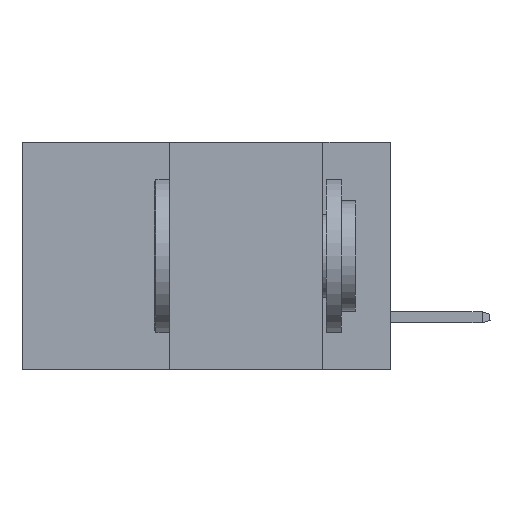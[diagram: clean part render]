
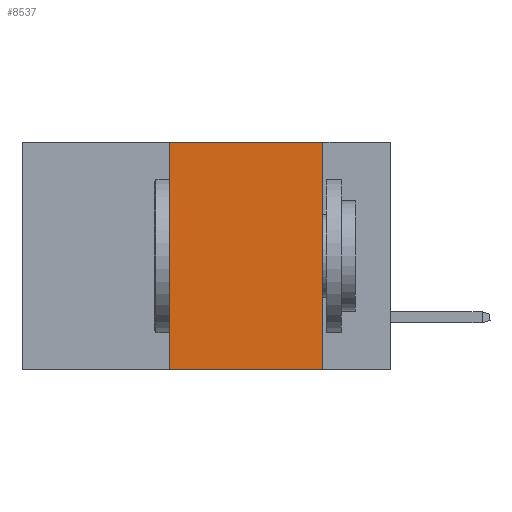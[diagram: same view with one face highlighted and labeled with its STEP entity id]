
A CAD part, left-side view. The second image highlights one B-rep face of the part: STEP entity #8537.
In plain terms, the highlighted planar face has unit normal (-1, 0, 0).
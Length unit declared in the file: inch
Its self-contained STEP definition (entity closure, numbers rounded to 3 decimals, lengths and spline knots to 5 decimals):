
#72 = VECTOR ( 'NONE', #18156, 39.37008 ) ;
#567 = VECTOR ( 'NONE', #1332, 39.37008 ) ;
#1215 = LINE ( 'NONE', #9681, #567 ) ;
#1332 = DIRECTION ( 'NONE',  ( 0., 0., -1. ) ) ;
#2672 = VECTOR ( 'NONE', #10832, 39.37008 ) ;
#2818 = DIRECTION ( 'NONE',  ( 0., -1., 0. ) ) ;
#4038 = ORIENTED_EDGE ( 'NONE', *, *, #9421, .F. ) ;
#4686 = ORIENTED_EDGE ( 'NONE', *, *, #11872, .F. ) ;
#4957 = LINE ( 'NONE', #16290, #72 ) ;
#5154 = VERTEX_POINT ( 'NONE', #15504 ) ;
#6317 = FACE_OUTER_BOUND ( 'NONE', #16492, .T. ) ;
#6521 = CARTESIAN_POINT ( 'NONE',  ( 0., 0.36, 0. ) ) ;
#6741 = CARTESIAN_POINT ( 'NONE',  ( 0., 0.6, -0.37 ) ) ;
#7179 = DIRECTION ( 'NONE',  ( 0., 0., -1. ) ) ;
#7308 = ORIENTED_EDGE ( 'NONE', *, *, #20778, .T. ) ;
#7364 = CARTESIAN_POINT ( 'NONE',  ( 0., 0.36, -0.37 ) ) ;
#8204 = LINE ( 'NONE', #6521, #2672 ) ;
#8537 = ADVANCED_FACE ( 'NONE', ( #6317 ), #19469, .F. ) ;
#9421 = EDGE_CURVE ( 'NONE', #26366, #26115, #8204, .T. ) ;
#9681 = CARTESIAN_POINT ( 'NONE',  ( 0., 0.11, 0. ) ) ;
#10832 = DIRECTION ( 'NONE',  ( 0., 0., 1. ) ) ;
#11872 = EDGE_CURVE ( 'NONE', #17773, #5154, #1215, .T. ) ;
#13207 = CARTESIAN_POINT ( 'NONE',  ( 0., 0.11, 0. ) ) ;
#13343 = CARTESIAN_POINT ( 'NONE',  ( 0., 0.6, 0. ) ) ;
#13422 = DIRECTION ( 'NONE',  ( 1., 0., 0. ) ) ;
#15504 = CARTESIAN_POINT ( 'NONE',  ( 0., 0.11, -0.37 ) ) ;
#15618 = AXIS2_PLACEMENT_3D ( 'NONE', #13343, #13422, #7179 ) ;
#15745 = ORIENTED_EDGE ( 'NONE', *, *, #22935, .F. ) ;
#16290 = CARTESIAN_POINT ( 'NONE',  ( 0., 0.6, 0. ) ) ;
#16492 = EDGE_LOOP ( 'NONE', ( #4686, #15745, #4038, #7308 ) ) ;
#17773 = VERTEX_POINT ( 'NONE', #13207 ) ;
#18156 = DIRECTION ( 'NONE',  ( 0., -1., 0. ) ) ;
#19469 = PLANE ( 'NONE',  #15618 ) ;
#20778 = EDGE_CURVE ( 'NONE', #26366, #5154, #24578, .T. ) ;
#22935 = EDGE_CURVE ( 'NONE', #26115, #17773, #4957, .T. ) ;
#23244 = VECTOR ( 'NONE', #2818, 39.37008 ) ;
#24578 = LINE ( 'NONE', #6741, #23244 ) ;
#25830 = CARTESIAN_POINT ( 'NONE',  ( 0., 0.36, 0. ) ) ;
#26115 = VERTEX_POINT ( 'NONE', #25830 ) ;
#26366 = VERTEX_POINT ( 'NONE', #7364 ) ;
